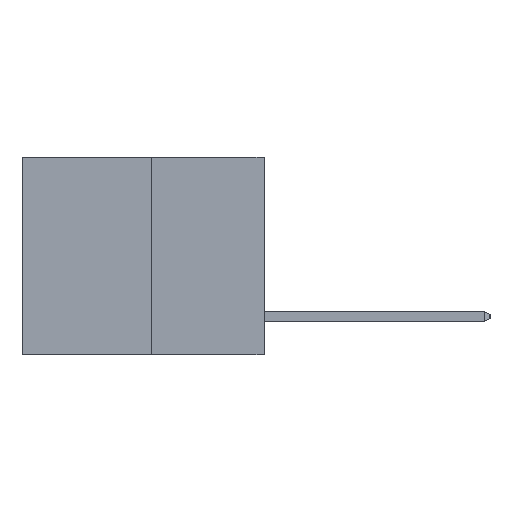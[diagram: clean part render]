
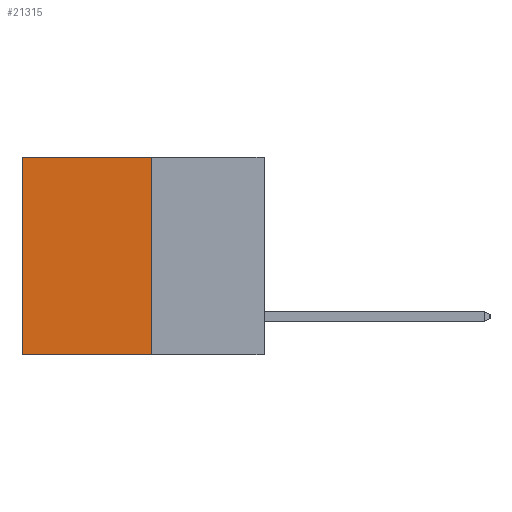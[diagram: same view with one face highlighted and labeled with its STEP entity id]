
A CAD part, left-side view. The second image highlights one B-rep face of the part: STEP entity #21315.
In plain terms, the highlighted planar face has unit normal (-1, 0, 0).
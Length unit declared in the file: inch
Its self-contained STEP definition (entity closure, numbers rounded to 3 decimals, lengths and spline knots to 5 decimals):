
#456 = DIRECTION ( 'NONE',  ( 0., 0., -1. ) ) ;
#702 = PLANE ( 'NONE',  #17107 ) ;
#1798 = VERTEX_POINT ( 'NONE', #24084 ) ;
#1944 = VERTEX_POINT ( 'NONE', #14735 ) ;
#2315 = VECTOR ( 'NONE', #11952, 39.37008 ) ;
#2968 = VERTEX_POINT ( 'NONE', #10569 ) ;
#4185 = CARTESIAN_POINT ( 'NONE',  ( 0.3165, 0.28, 0. ) ) ;
#5760 = EDGE_LOOP ( 'NONE', ( #21393, #12813, #23757, #25049 ) ) ;
#5992 = EDGE_CURVE ( 'NONE', #1944, #23659, #20390, .T. ) ;
#7942 = CARTESIAN_POINT ( 'NONE',  ( 0.3165, 0.28, -0.49 ) ) ;
#8108 = DIRECTION ( 'NONE',  ( 0., 0., -1. ) ) ;
#9727 = CARTESIAN_POINT ( 'NONE',  ( 0.3165, 0.6, -0.49 ) ) ;
#10569 = CARTESIAN_POINT ( 'NONE',  ( 0.3165, 0.28, 0. ) ) ;
#10572 = EDGE_CURVE ( 'NONE', #2968, #1798, #12672, .T. ) ;
#11952 = DIRECTION ( 'NONE',  ( 0., 1., 0. ) ) ;
#12278 = EDGE_CURVE ( 'NONE', #2968, #1944, #21105, .T. ) ;
#12672 = LINE ( 'NONE', #4185, #2315 ) ;
#12813 = ORIENTED_EDGE ( 'NONE', *, *, #5992, .F. ) ;
#14735 = CARTESIAN_POINT ( 'NONE',  ( 0.3165, 0.28, -0.49 ) ) ;
#14742 = FACE_OUTER_BOUND ( 'NONE', #5760, .T. ) ;
#15342 = VECTOR ( 'NONE', #23700, 39.37008 ) ;
#15845 = EDGE_CURVE ( 'NONE', #1798, #23659, #20484, .T. ) ;
#16804 = CARTESIAN_POINT ( 'NONE',  ( 0.3165, 0.28, -0.49 ) ) ;
#17107 = AXIS2_PLACEMENT_3D ( 'NONE', #21746, #23737, #456 ) ;
#17289 = CARTESIAN_POINT ( 'NONE',  ( 0.3165, 0.6, -0.49 ) ) ;
#20390 = LINE ( 'NONE', #16804, #20981 ) ;
#20484 = LINE ( 'NONE', #9727, #21966 ) ;
#20981 = VECTOR ( 'NONE', #24675, 39.37008 ) ;
#21105 = LINE ( 'NONE', #7942, #15342 ) ;
#21315 = ADVANCED_FACE ( 'NONE', ( #14742 ), #702, .F. ) ;
#21393 = ORIENTED_EDGE ( 'NONE', *, *, #15845, .T. ) ;
#21746 = CARTESIAN_POINT ( 'NONE',  ( 0.3165, 0.28, -0.49 ) ) ;
#21966 = VECTOR ( 'NONE', #8108, 39.37008 ) ;
#23659 = VERTEX_POINT ( 'NONE', #17289 ) ;
#23700 = DIRECTION ( 'NONE',  ( 0., 0., -1. ) ) ;
#23737 = DIRECTION ( 'NONE',  ( 1., 0., 0. ) ) ;
#23757 = ORIENTED_EDGE ( 'NONE', *, *, #12278, .F. ) ;
#24084 = CARTESIAN_POINT ( 'NONE',  ( 0.3165, 0.6, 0. ) ) ;
#24675 = DIRECTION ( 'NONE',  ( 0., 1., 0. ) ) ;
#25049 = ORIENTED_EDGE ( 'NONE', *, *, #10572, .T. ) ;
